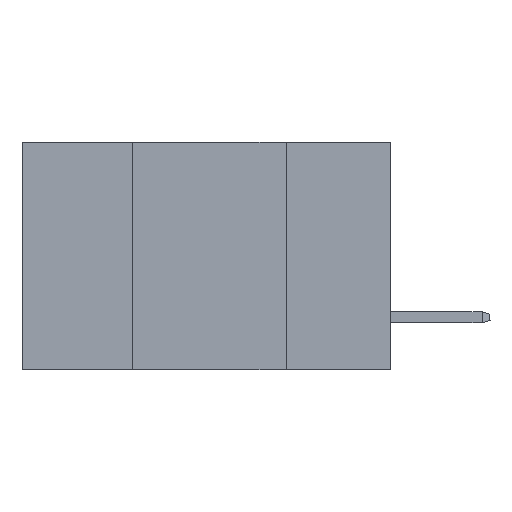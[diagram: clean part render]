
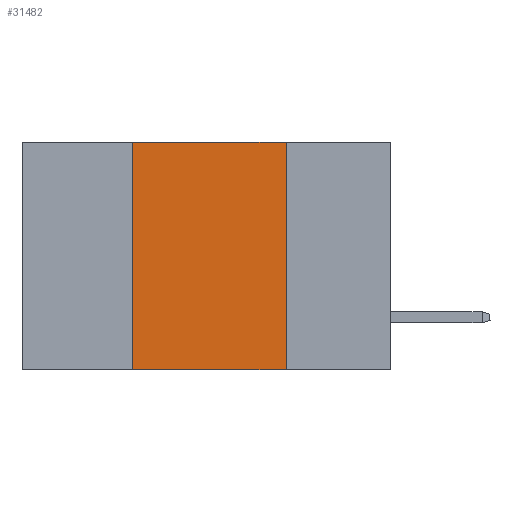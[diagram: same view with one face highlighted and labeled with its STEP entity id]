
A CAD part, left-side view. The second image highlights one B-rep face of the part: STEP entity #31482.
In plain terms, the highlighted planar face has unit normal (-1, 0, 0).
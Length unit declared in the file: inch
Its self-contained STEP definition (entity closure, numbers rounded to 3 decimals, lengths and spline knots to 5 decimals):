
#364 = ORIENTED_EDGE ( 'NONE', *, *, #14198, .F. ) ;
#394 = LINE ( 'NONE', #7082, #31274 ) ;
#2467 = CARTESIAN_POINT ( 'NONE',  ( 0., 0.17, -0.37 ) ) ;
#2880 = CARTESIAN_POINT ( 'NONE',  ( 0., 0.17, 0. ) ) ;
#3310 = CARTESIAN_POINT ( 'NONE',  ( 0., 0.42, -0.37 ) ) ;
#3345 = LINE ( 'NONE', #2880, #7662 ) ;
#4084 = VERTEX_POINT ( 'NONE', #3310 ) ;
#6607 = VERTEX_POINT ( 'NONE', #12672 ) ;
#7082 = CARTESIAN_POINT ( 'NONE',  ( 0., 0.6, -0.37 ) ) ;
#7662 = VECTOR ( 'NONE', #7704, 39.37008 ) ;
#7704 = DIRECTION ( 'NONE',  ( 0., 0., -1. ) ) ;
#8592 = DIRECTION ( 'NONE',  ( 0., 0., -1. ) ) ;
#8929 = LINE ( 'NONE', #22248, #27230 ) ;
#10993 = PLANE ( 'NONE',  #22772 ) ;
#12438 = DIRECTION ( 'NONE',  ( 0., -1., 0. ) ) ;
#12672 = CARTESIAN_POINT ( 'NONE',  ( 0., 0.42, 0. ) ) ;
#14198 = EDGE_CURVE ( 'NONE', #4084, #6607, #29752, .T. ) ;
#16052 = EDGE_CURVE ( 'NONE', #4084, #31299, #394, .T. ) ;
#16102 = CARTESIAN_POINT ( 'NONE',  ( 0., 0.6, 0. ) ) ;
#17439 = EDGE_CURVE ( 'NONE', #6607, #29281, #8929, .T. ) ;
#19719 = DIRECTION ( 'NONE',  ( 0., -1., 0. ) ) ;
#21030 = EDGE_CURVE ( 'NONE', #29281, #31299, #3345, .T. ) ;
#22248 = CARTESIAN_POINT ( 'NONE',  ( 0., 0.6, 0. ) ) ;
#22772 = AXIS2_PLACEMENT_3D ( 'NONE', #16102, #30288, #8592 ) ;
#22776 = VECTOR ( 'NONE', #27908, 39.37008 ) ;
#23372 = FACE_OUTER_BOUND ( 'NONE', #28651, .T. ) ;
#24652 = CARTESIAN_POINT ( 'NONE',  ( 0., 0.17, 0. ) ) ;
#25091 = CARTESIAN_POINT ( 'NONE',  ( 0., 0.42, 0. ) ) ;
#27230 = VECTOR ( 'NONE', #19719, 39.37008 ) ;
#27293 = ORIENTED_EDGE ( 'NONE', *, *, #21030, .F. ) ;
#27908 = DIRECTION ( 'NONE',  ( 0., 0., 1. ) ) ;
#27918 = ORIENTED_EDGE ( 'NONE', *, *, #16052, .T. ) ;
#28651 = EDGE_LOOP ( 'NONE', ( #27293, #30896, #364, #27918 ) ) ;
#29281 = VERTEX_POINT ( 'NONE', #24652 ) ;
#29752 = LINE ( 'NONE', #25091, #22776 ) ;
#30288 = DIRECTION ( 'NONE',  ( 1., 0., 0. ) ) ;
#30896 = ORIENTED_EDGE ( 'NONE', *, *, #17439, .F. ) ;
#31274 = VECTOR ( 'NONE', #12438, 39.37008 ) ;
#31299 = VERTEX_POINT ( 'NONE', #2467 ) ;
#31482 = ADVANCED_FACE ( 'NONE', ( #23372 ), #10993, .F. ) ;
